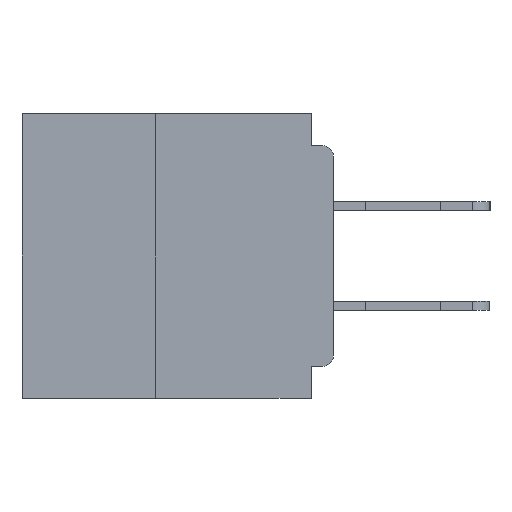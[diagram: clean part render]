
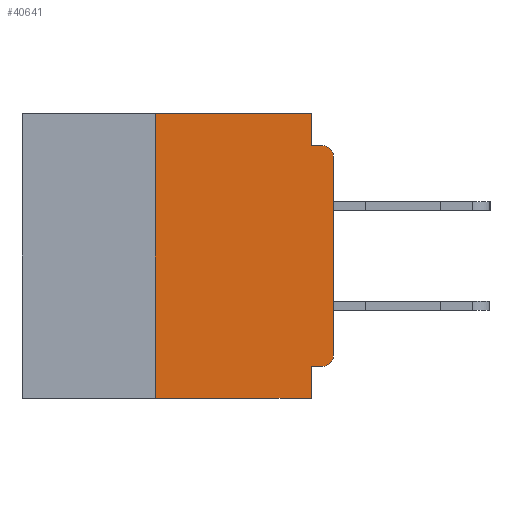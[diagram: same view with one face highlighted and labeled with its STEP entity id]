
A CAD part, left-side view. The second image highlights one B-rep face of the part: STEP entity #40641.
In plain terms, the highlighted planar face has unit normal (-1, 0, 0).
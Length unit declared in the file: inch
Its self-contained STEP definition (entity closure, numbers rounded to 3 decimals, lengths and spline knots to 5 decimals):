
#613 = CIRCLE ( 'NONE', #19033, 0.015 ) ;
#1872 = EDGE_LOOP ( 'NONE', ( #10101, #19147, #37380, #30419, #39577, #15479, #24489, #33643, #18646, #30974 ) ) ;
#3866 = EDGE_CURVE ( 'NONE', #11925, #24264, #38115, .T. ) ;
#4039 = CARTESIAN_POINT ( 'NONE',  ( 0., 0.015, -0.045 ) ) ;
#4858 = CARTESIAN_POINT ( 'NONE',  ( 0., 0.031, -0.355 ) ) ;
#4955 = LINE ( 'NONE', #20717, #31215 ) ;
#4960 = CARTESIAN_POINT ( 'NONE',  ( 0., 0.25, -0.4 ) ) ;
#4989 = DIRECTION ( 'NONE',  ( 0., -1., 0. ) ) ;
#5469 = CARTESIAN_POINT ( 'NONE',  ( 0., 0.015, -0.34 ) ) ;
#6503 = CARTESIAN_POINT ( 'NONE',  ( 0., 0.437, 0. ) ) ;
#6785 = CARTESIAN_POINT ( 'NONE',  ( 0., 0.031, 0. ) ) ;
#6814 = AXIS2_PLACEMENT_3D ( 'NONE', #6503, #30466, #9993 ) ;
#8654 = CARTESIAN_POINT ( 'NONE',  ( 0., 0., 0. ) ) ;
#8935 = DIRECTION ( 'NONE',  ( 0., 0., -1. ) ) ;
#9098 = CARTESIAN_POINT ( 'NONE',  ( 0., 0.015, -0.06 ) ) ;
#9431 = EDGE_CURVE ( 'NONE', #29188, #13946, #15847, .T. ) ;
#9530 = CARTESIAN_POINT ( 'NONE',  ( 0., 0.031, -0.4 ) ) ;
#9993 = DIRECTION ( 'NONE',  ( 0., 0., -1. ) ) ;
#10101 = ORIENTED_EDGE ( 'NONE', *, *, #44311, .T. ) ;
#10275 = CARTESIAN_POINT ( 'NONE',  ( 0., 0.437, -0.4 ) ) ;
#10453 = VECTOR ( 'NONE', #12113, 39.37008 ) ;
#11094 = EDGE_CURVE ( 'NONE', #41590, #32281, #613, .T. ) ;
#11363 = EDGE_CURVE ( 'NONE', #29461, #13946, #17244, .T. ) ;
#11925 = VERTEX_POINT ( 'NONE', #16773 ) ;
#12113 = DIRECTION ( 'NONE',  ( 0., 0., 1. ) ) ;
#12574 = DIRECTION ( 'NONE',  ( 0., 0., -1. ) ) ;
#13946 = VERTEX_POINT ( 'NONE', #36858 ) ;
#15479 = ORIENTED_EDGE ( 'NONE', *, *, #15851, .F. ) ;
#15847 = LINE ( 'NONE', #9530, #30783 ) ;
#15851 = EDGE_CURVE ( 'NONE', #29461, #32853, #39010, .T. ) ;
#16773 = CARTESIAN_POINT ( 'NONE',  ( 0., 0.031, -0.045 ) ) ;
#17244 = LINE ( 'NONE', #10275, #26303 ) ;
#17731 = CARTESIAN_POINT ( 'NONE',  ( 0., 0.031, 0. ) ) ;
#18474 = VERTEX_POINT ( 'NONE', #17731 ) ;
#18646 = ORIENTED_EDGE ( 'NONE', *, *, #40046, .F. ) ;
#18804 = VECTOR ( 'NONE', #29301, 39.37008 ) ;
#19033 = AXIS2_PLACEMENT_3D ( 'NONE', #5469, #29416, #8935 ) ;
#19147 = ORIENTED_EDGE ( 'NONE', *, *, #38582, .T. ) ;
#20405 = VERTEX_POINT ( 'NONE', #34467 ) ;
#20717 = CARTESIAN_POINT ( 'NONE',  ( 0., 0., -0.355 ) ) ;
#22654 = EDGE_CURVE ( 'NONE', #18474, #11925, #23893, .T. ) ;
#22841 = VECTOR ( 'NONE', #41109, 39.37008 ) ;
#23893 = LINE ( 'NONE', #6785, #22841 ) ;
#24166 = DIRECTION ( 'NONE',  ( 0., 1., 0. ) ) ;
#24264 = VERTEX_POINT ( 'NONE', #4039 ) ;
#24489 = ORIENTED_EDGE ( 'NONE', *, *, #11363, .T. ) ;
#24679 = FACE_OUTER_BOUND ( 'NONE', #1872, .T. ) ;
#25432 = DIRECTION ( 'NONE',  ( 0., 0., 1. ) ) ;
#26303 = VECTOR ( 'NONE', #30722, 39.37008 ) ;
#28189 = CARTESIAN_POINT ( 'NONE',  ( 0., 0.25, 0. ) ) ;
#29188 = VERTEX_POINT ( 'NONE', #4858 ) ;
#29301 = DIRECTION ( 'NONE',  ( 0., -1., 0. ) ) ;
#29356 = CARTESIAN_POINT ( 'NONE',  ( 0., 0., -0.045 ) ) ;
#29416 = DIRECTION ( 'NONE',  ( -1., 0., 0. ) ) ;
#29461 = VERTEX_POINT ( 'NONE', #30007 ) ;
#29541 = CARTESIAN_POINT ( 'NONE',  ( 0., 0.015, -0.355 ) ) ;
#30007 = CARTESIAN_POINT ( 'NONE',  ( 0., 0.25, -0.4 ) ) ;
#30419 = ORIENTED_EDGE ( 'NONE', *, *, #22654, .F. ) ;
#30466 = DIRECTION ( 'NONE',  ( 1., 0., 0. ) ) ;
#30722 = DIRECTION ( 'NONE',  ( 0., -1., 0. ) ) ;
#30783 = VECTOR ( 'NONE', #43752, 39.37008 ) ;
#30974 = ORIENTED_EDGE ( 'NONE', *, *, #11094, .T. ) ;
#31215 = VECTOR ( 'NONE', #24166, 39.37008 ) ;
#32281 = VERTEX_POINT ( 'NONE', #37014 ) ;
#32853 = VERTEX_POINT ( 'NONE', #28189 ) ;
#33005 = DIRECTION ( 'NONE',  ( -1., 0., 0. ) ) ;
#33643 = ORIENTED_EDGE ( 'NONE', *, *, #9431, .F. ) ;
#34467 = CARTESIAN_POINT ( 'NONE',  ( 0., 0., -0.06 ) ) ;
#34748 = EDGE_CURVE ( 'NONE', #32853, #18474, #38882, .T. ) ;
#35032 = CIRCLE ( 'NONE', #40377, 0.015 ) ;
#35846 = CARTESIAN_POINT ( 'NONE',  ( 0., 0.437, 0. ) ) ;
#36654 = LINE ( 'NONE', #8654, #10453 ) ;
#36838 = VECTOR ( 'NONE', #25432, 39.37008 ) ;
#36858 = CARTESIAN_POINT ( 'NONE',  ( 0., 0.031, -0.4 ) ) ;
#37014 = CARTESIAN_POINT ( 'NONE',  ( 0., 0., -0.34 ) ) ;
#37380 = ORIENTED_EDGE ( 'NONE', *, *, #3866, .F. ) ;
#37794 = VECTOR ( 'NONE', #4989, 39.37008 ) ;
#38115 = LINE ( 'NONE', #29356, #18804 ) ;
#38582 = EDGE_CURVE ( 'NONE', #20405, #24264, #35032, .T. ) ;
#38882 = LINE ( 'NONE', #35846, #37794 ) ;
#39010 = LINE ( 'NONE', #4960, #36838 ) ;
#39577 = ORIENTED_EDGE ( 'NONE', *, *, #34748, .F. ) ;
#40046 = EDGE_CURVE ( 'NONE', #41590, #29188, #4955, .T. ) ;
#40377 = AXIS2_PLACEMENT_3D ( 'NONE', #9098, #33005, #12574 ) ;
#40641 = ADVANCED_FACE ( 'NONE', ( #24679 ), #40692, .F. ) ;
#40692 = PLANE ( 'NONE',  #6814 ) ;
#41109 = DIRECTION ( 'NONE',  ( 0., 0., -1. ) ) ;
#41590 = VERTEX_POINT ( 'NONE', #29541 ) ;
#43752 = DIRECTION ( 'NONE',  ( 0., 0., -1. ) ) ;
#44311 = EDGE_CURVE ( 'NONE', #32281, #20405, #36654, .T. ) ;
